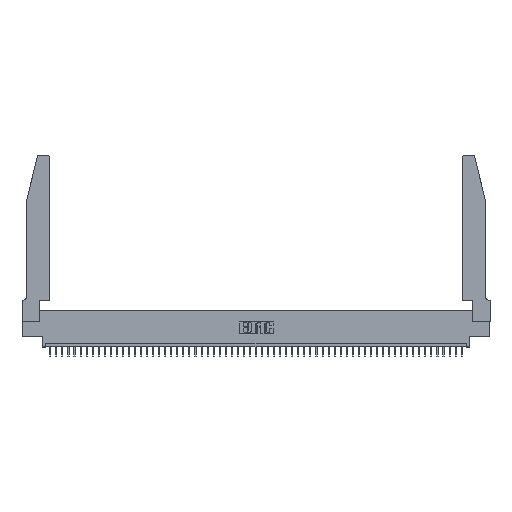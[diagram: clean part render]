
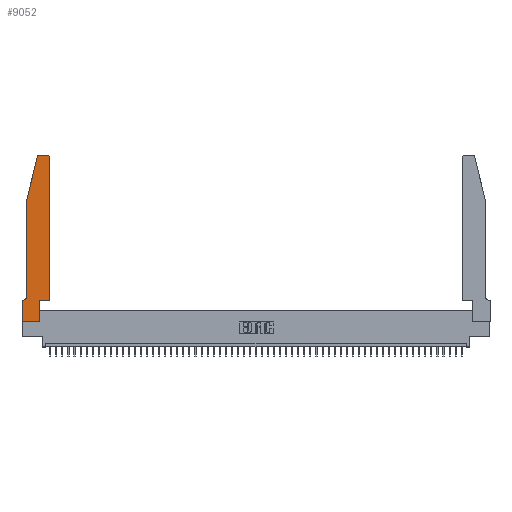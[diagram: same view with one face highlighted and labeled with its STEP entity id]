
A CAD part, top view. The second image highlights one B-rep face of the part: STEP entity #9052.
In plain terms, the highlighted planar face has unit normal (0, 0, 1).
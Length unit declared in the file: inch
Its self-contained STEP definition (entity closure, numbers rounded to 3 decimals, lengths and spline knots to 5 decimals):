
#209 = ORIENTED_EDGE ( 'NONE', *, *, #9934, .T. ) ;
#386 = DIRECTION ( 'NONE',  ( -1., 0., 0. ) ) ;
#388 = LINE ( 'NONE', #1647, #8167 ) ;
#1163 = CARTESIAN_POINT ( 'NONE',  ( 0.2865, 0.35, 0.37 ) ) ;
#1647 = CARTESIAN_POINT ( 'NONE',  ( 0.4505, 0.35, 0.37 ) ) ;
#2163 = VERTEX_POINT ( 'NONE', #37958 ) ;
#2417 = VERTEX_POINT ( 'NONE', #47710 ) ;
#2642 = CARTESIAN_POINT ( 'NONE',  ( 0., 0., 0.37 ) ) ;
#2826 = CARTESIAN_POINT ( 'NONE',  ( 0.0755, 2., 0.37 ) ) ;
#3597 = DIRECTION ( 'NONE',  ( 1., 0., 0. ) ) ;
#4371 = LINE ( 'NONE', #20003, #27486 ) ;
#4501 = CIRCLE ( 'NONE', #40226, 0.03 ) ;
#4733 = DIRECTION ( 'NONE',  ( 0., 0., -1. ) ) ;
#5014 = LINE ( 'NONE', #1163, #17827 ) ;
#5234 = FACE_OUTER_BOUND ( 'NONE', #28111, .T. ) ;
#5648 = EDGE_CURVE ( 'NONE', #49832, #2163, #31988, .T. ) ;
#7179 = ORIENTED_EDGE ( 'NONE', *, *, #5648, .T. ) ;
#7580 = DIRECTION ( 'NONE',  ( -1., 0., 0. ) ) ;
#8143 = CARTESIAN_POINT ( 'NONE',  ( 0.4205, 2.72, 0.37 ) ) ;
#8167 = VECTOR ( 'NONE', #34498, 39.37008 ) ;
#8319 = DIRECTION ( 'NONE',  ( 1., 0., 0. ) ) ;
#8623 = CARTESIAN_POINT ( 'NONE',  ( 0., 0.35, 0.37 ) ) ;
#8821 = DIRECTION ( 'NONE',  ( -1., 0., 0. ) ) ;
#9052 = ADVANCED_FACE ( 'NONE', ( #5234 ), #34601, .T. ) ;
#9851 = AXIS2_PLACEMENT_3D ( 'NONE', #16938, #4733, #386 ) ;
#9934 = EDGE_CURVE ( 'NONE', #27595, #17698, #36573, .T. ) ;
#10733 = EDGE_CURVE ( 'NONE', #16686, #24058, #4371, .T. ) ;
#10744 = DIRECTION ( 'NONE',  ( 0., -1., 0. ) ) ;
#10852 = VERTEX_POINT ( 'NONE', #21711 ) ;
#11310 = DIRECTION ( 'NONE',  ( 0., -1., 0. ) ) ;
#12199 = VECTOR ( 'NONE', #7580, 39.37008 ) ;
#12549 = CARTESIAN_POINT ( 'NONE',  ( 0.0755, 0.42, 0.37 ) ) ;
#13405 = ORIENTED_EDGE ( 'NONE', *, *, #37928, .T. ) ;
#13432 = VECTOR ( 'NONE', #8821, 39.37008 ) ;
#13714 = VERTEX_POINT ( 'NONE', #8623 ) ;
#15921 = ORIENTED_EDGE ( 'NONE', *, *, #17599, .T. ) ;
#16151 = ORIENTED_EDGE ( 'NONE', *, *, #28402, .T. ) ;
#16686 = VERTEX_POINT ( 'NONE', #18968 ) ;
#16938 = CARTESIAN_POINT ( 'NONE',  ( 0.0055, 0.42, 0.37 ) ) ;
#17338 = DIRECTION ( 'NONE',  ( 1., 0., 0. ) ) ;
#17599 = EDGE_CURVE ( 'NONE', #34975, #13714, #40396, .T. ) ;
#17698 = VERTEX_POINT ( 'NONE', #21566 ) ;
#17827 = VECTOR ( 'NONE', #34193, 39.37008 ) ;
#17886 = VECTOR ( 'NONE', #52373, 39.37008 ) ;
#17920 = CARTESIAN_POINT ( 'NONE',  ( 0.25487, 2.72718, 0.37 ) ) ;
#18254 = ORIENTED_EDGE ( 'NONE', *, *, #48208, .T. ) ;
#18279 = DIRECTION ( 'NONE',  ( 0., 0., 1. ) ) ;
#18554 = EDGE_CURVE ( 'NONE', #24058, #27595, #5014, .T. ) ;
#18968 = CARTESIAN_POINT ( 'NONE',  ( 0., 0., 0.37 ) ) ;
#19646 = DIRECTION ( 'NONE',  ( 1., 0., 0. ) ) ;
#20003 = CARTESIAN_POINT ( 'NONE',  ( 0., 0., 0.37 ) ) ;
#20632 = CIRCLE ( 'NONE', #33726, 0.03 ) ;
#20647 = ORIENTED_EDGE ( 'NONE', *, *, #18554, .T. ) ;
#21451 = VECTOR ( 'NONE', #11310, 39.37008 ) ;
#21492 = CARTESIAN_POINT ( 'NONE',  ( 0.284, 2.72, 0.37 ) ) ;
#21566 = CARTESIAN_POINT ( 'NONE',  ( 0.4505, 0.35, 0.37 ) ) ;
#21711 = CARTESIAN_POINT ( 'NONE',  ( 0.284, 2.75, 0.37 ) ) ;
#24058 = VERTEX_POINT ( 'NONE', #43941 ) ;
#24803 = EDGE_CURVE ( 'NONE', #2417, #10852, #44977, .T. ) ;
#25816 = CIRCLE ( 'NONE', #9851, 0.07 ) ;
#27486 = VECTOR ( 'NONE', #19646, 39.37008 ) ;
#27595 = VERTEX_POINT ( 'NONE', #39524 ) ;
#27635 = CARTESIAN_POINT ( 'NONE',  ( 0.0755, 2., 0.37 ) ) ;
#28111 = EDGE_LOOP ( 'NONE', ( #45796, #37014, #7179, #16151, #13405, #15921, #18254, #31873, #20647, #209, #34423, #33684 ) ) ;
#28402 = EDGE_CURVE ( 'NONE', #2163, #46397, #43278, .T. ) ;
#29762 = AXIS2_PLACEMENT_3D ( 'NONE', #42891, #18279, #47043 ) ;
#31462 = VECTOR ( 'NONE', #3597, 39.37008 ) ;
#31465 = EDGE_CURVE ( 'NONE', #10852, #49832, #4501, .T. ) ;
#31799 = CARTESIAN_POINT ( 'NONE',  ( 0.0055, 0.35, 0.37 ) ) ;
#31873 = ORIENTED_EDGE ( 'NONE', *, *, #10733, .T. ) ;
#31988 = LINE ( 'NONE', #2826, #17886 ) ;
#33263 = EDGE_CURVE ( 'NONE', #17698, #48836, #388, .T. ) ;
#33568 = CARTESIAN_POINT ( 'NONE',  ( 0.0755, 0.35, 0.37 ) ) ;
#33684 = ORIENTED_EDGE ( 'NONE', *, *, #43586, .T. ) ;
#33726 = AXIS2_PLACEMENT_3D ( 'NONE', #8143, #44594, #8319 ) ;
#34193 = DIRECTION ( 'NONE',  ( 0., 1., 0. ) ) ;
#34355 = CARTESIAN_POINT ( 'NONE',  ( 0.4505, 2.72, 0.37 ) ) ;
#34423 = ORIENTED_EDGE ( 'NONE', *, *, #33263, .T. ) ;
#34498 = DIRECTION ( 'NONE',  ( 0., 1., 0. ) ) ;
#34601 = PLANE ( 'NONE',  #29762 ) ;
#34975 = VERTEX_POINT ( 'NONE', #31799 ) ;
#36573 = LINE ( 'NONE', #37115, #31462 ) ;
#37014 = ORIENTED_EDGE ( 'NONE', *, *, #31465, .T. ) ;
#37115 = CARTESIAN_POINT ( 'NONE',  ( 0.4505, 0.35, 0.37 ) ) ;
#37928 = EDGE_CURVE ( 'NONE', #46397, #34975, #25816, .T. ) ;
#37958 = CARTESIAN_POINT ( 'NONE',  ( 0.0755, 2., 0.37 ) ) ;
#38298 = DIRECTION ( 'NONE',  ( 0., 0., 1. ) ) ;
#39524 = CARTESIAN_POINT ( 'NONE',  ( 0.2865, 0.35, 0.37 ) ) ;
#40226 = AXIS2_PLACEMENT_3D ( 'NONE', #21492, #38298, #17338 ) ;
#40396 = LINE ( 'NONE', #33568, #13432 ) ;
#42891 = CARTESIAN_POINT ( 'NONE',  ( 0., 0.35, 0.37 ) ) ;
#43278 = LINE ( 'NONE', #27635, #21451 ) ;
#43319 = VECTOR ( 'NONE', #10744, 39.37008 ) ;
#43586 = EDGE_CURVE ( 'NONE', #48836, #2417, #20632, .T. ) ;
#43941 = CARTESIAN_POINT ( 'NONE',  ( 0.2865, 0., 0.37 ) ) ;
#44409 = CARTESIAN_POINT ( 'NONE',  ( 0.2605, 2.75, 0.37 ) ) ;
#44594 = DIRECTION ( 'NONE',  ( 0., 0., 1. ) ) ;
#44977 = LINE ( 'NONE', #44409, #12199 ) ;
#45796 = ORIENTED_EDGE ( 'NONE', *, *, #24803, .T. ) ;
#46397 = VERTEX_POINT ( 'NONE', #12549 ) ;
#47043 = DIRECTION ( 'NONE',  ( 1., 0., 0. ) ) ;
#47710 = CARTESIAN_POINT ( 'NONE',  ( 0.4205, 2.75, 0.37 ) ) ;
#48208 = EDGE_CURVE ( 'NONE', #13714, #16686, #50392, .T. ) ;
#48836 = VERTEX_POINT ( 'NONE', #34355 ) ;
#49832 = VERTEX_POINT ( 'NONE', #17920 ) ;
#50392 = LINE ( 'NONE', #2642, #43319 ) ;
#52373 = DIRECTION ( 'NONE',  ( -0.239, -0.971, 0. ) ) ;
